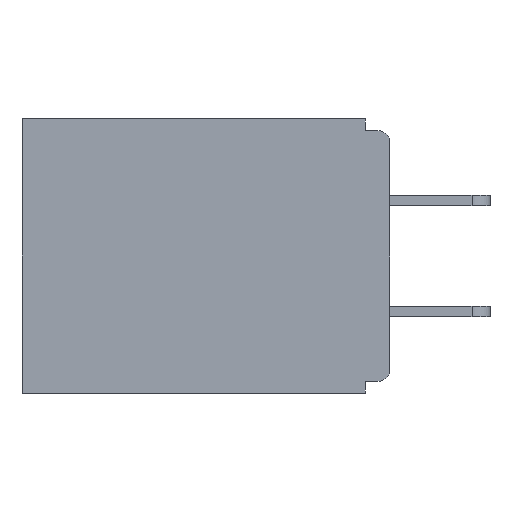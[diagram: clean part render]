
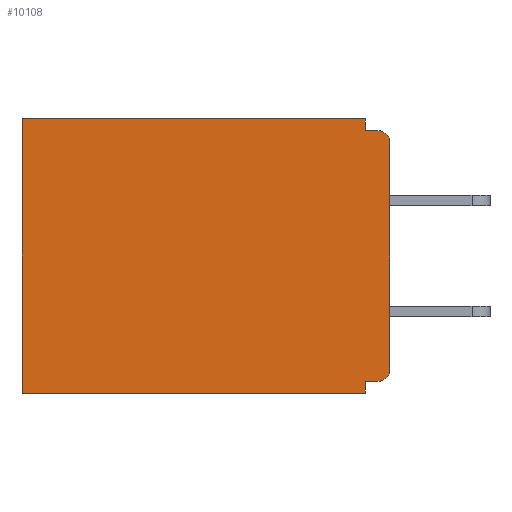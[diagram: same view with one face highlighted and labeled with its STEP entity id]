
A CAD part, left-side view. The second image highlights one B-rep face of the part: STEP entity #10108.
In plain terms, the highlighted planar face has unit normal (-1, 0, 0).
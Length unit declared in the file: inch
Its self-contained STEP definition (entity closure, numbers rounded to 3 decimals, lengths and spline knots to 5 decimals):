
#109 = VERTEX_POINT ( 'NONE', #1873 ) ;
#428 = ORIENTED_EDGE ( 'NONE', *, *, #12479, .F. ) ;
#603 = CARTESIAN_POINT ( 'NONE',  ( 0.298, 0.015, -0.313 ) ) ;
#623 = LINE ( 'NONE', #15823, #2158 ) ;
#644 = LINE ( 'NONE', #12943, #10087 ) ;
#671 = CARTESIAN_POINT ( 'NONE',  ( 0.298, 0.015, -0.015 ) ) ;
#1138 = DIRECTION ( 'NONE',  ( 0., 0., -1. ) ) ;
#1159 = DIRECTION ( 'NONE',  ( 0., 1., 0. ) ) ;
#1163 = VERTEX_POINT ( 'NONE', #1696 ) ;
#1213 = CARTESIAN_POINT ( 'NONE',  ( 0.298, 0., -0.328 ) ) ;
#1373 = VERTEX_POINT ( 'NONE', #3288 ) ;
#1416 = EDGE_CURVE ( 'NONE', #12056, #1445, #12308, .T. ) ;
#1445 = VERTEX_POINT ( 'NONE', #14474 ) ;
#1696 = CARTESIAN_POINT ( 'NONE',  ( 0.298, 0.031, -0.328 ) ) ;
#1727 = DIRECTION ( 'NONE',  ( 0., -1., 0. ) ) ;
#1795 = ORIENTED_EDGE ( 'NONE', *, *, #8183, .F. ) ;
#1815 = VECTOR ( 'NONE', #4954, 39.37008 ) ;
#1835 = LINE ( 'NONE', #6711, #13068 ) ;
#1873 = CARTESIAN_POINT ( 'NONE',  ( 0.298, 0.46, -0.343 ) ) ;
#2158 = VECTOR ( 'NONE', #14056, 39.37008 ) ;
#2245 = DIRECTION ( 'NONE',  ( 0., 0., -1. ) ) ;
#2521 = ORIENTED_EDGE ( 'NONE', *, *, #8639, .T. ) ;
#3025 = LINE ( 'NONE', #12281, #6350 ) ;
#3256 = LINE ( 'NONE', #7422, #12348 ) ;
#3288 = CARTESIAN_POINT ( 'NONE',  ( 0.298, 0.031, -0.015 ) ) ;
#3484 = CARTESIAN_POINT ( 'NONE',  ( 0.298, 0.015, -0.328 ) ) ;
#4926 = CARTESIAN_POINT ( 'NONE',  ( 0.298, 0.031, 0. ) ) ;
#4954 = DIRECTION ( 'NONE',  ( 0., 1., 0. ) ) ;
#5056 = VERTEX_POINT ( 'NONE', #15308 ) ;
#5442 = CARTESIAN_POINT ( 'NONE',  ( 0.298, 0.46, 0. ) ) ;
#5462 = ORIENTED_EDGE ( 'NONE', *, *, #12896, .F. ) ;
#5669 = EDGE_CURVE ( 'NONE', #13512, #1445, #3256, .T. ) ;
#5830 = DIRECTION ( 'NONE',  ( 0., 1., 0. ) ) ;
#6000 = DIRECTION ( 'NONE',  ( -1., 0., 0. ) ) ;
#6046 = AXIS2_PLACEMENT_3D ( 'NONE', #603, #9306, #13221 ) ;
#6350 = VECTOR ( 'NONE', #2245, 39.37008 ) ;
#6384 = AXIS2_PLACEMENT_3D ( 'NONE', #14860, #15900, #8569 ) ;
#6418 = ORIENTED_EDGE ( 'NONE', *, *, #7028, .F. ) ;
#6711 = CARTESIAN_POINT ( 'NONE',  ( 0.298, 0., -0.015 ) ) ;
#7028 = EDGE_CURVE ( 'NONE', #10719, #1373, #3025, .T. ) ;
#7046 = EDGE_LOOP ( 'NONE', ( #9855, #1795, #6418, #2521, #9861, #428, #12510, #5462, #11196, #9612 ) ) ;
#7422 = CARTESIAN_POINT ( 'NONE',  ( 0.298, 0., 0. ) ) ;
#7635 = CIRCLE ( 'NONE', #15856, 0.015 ) ;
#8183 = EDGE_CURVE ( 'NONE', #1373, #9419, #1835, .T. ) ;
#8259 = CARTESIAN_POINT ( 'NONE',  ( 0.298, 0., -0.343 ) ) ;
#8569 = DIRECTION ( 'NONE',  ( 0., 0., -1. ) ) ;
#8623 = VECTOR ( 'NONE', #5830, 39.37008 ) ;
#8639 = EDGE_CURVE ( 'NONE', #10719, #10470, #15396, .T. ) ;
#9102 = EDGE_CURVE ( 'NONE', #1163, #5056, #644, .T. ) ;
#9306 = DIRECTION ( 'NONE',  ( -1., 0., 0. ) ) ;
#9384 = VECTOR ( 'NONE', #1159, 39.37008 ) ;
#9419 = VERTEX_POINT ( 'NONE', #671 ) ;
#9420 = LINE ( 'NONE', #8259, #8623 ) ;
#9612 = ORIENTED_EDGE ( 'NONE', *, *, #5669, .F. ) ;
#9855 = ORIENTED_EDGE ( 'NONE', *, *, #12700, .T. ) ;
#9861 = ORIENTED_EDGE ( 'NONE', *, *, #11090, .T. ) ;
#10087 = VECTOR ( 'NONE', #14303, 39.37008 ) ;
#10108 = ADVANCED_FACE ( 'NONE', ( #14792 ), #13600, .F. ) ;
#10470 = VERTEX_POINT ( 'NONE', #5442 ) ;
#10719 = VERTEX_POINT ( 'NONE', #4926 ) ;
#11090 = EDGE_CURVE ( 'NONE', #10470, #109, #623, .T. ) ;
#11112 = CARTESIAN_POINT ( 'NONE',  ( 0.298, 0.015, -0.03 ) ) ;
#11196 = ORIENTED_EDGE ( 'NONE', *, *, #1416, .T. ) ;
#12056 = VERTEX_POINT ( 'NONE', #3484 ) ;
#12281 = CARTESIAN_POINT ( 'NONE',  ( 0.298, 0.031, -0.343 ) ) ;
#12308 = CIRCLE ( 'NONE', #6046, 0.015 ) ;
#12348 = VECTOR ( 'NONE', #16180, 39.37008 ) ;
#12479 = EDGE_CURVE ( 'NONE', #5056, #109, #9420, .T. ) ;
#12509 = CARTESIAN_POINT ( 'NONE',  ( 0.298, 0., 0. ) ) ;
#12510 = ORIENTED_EDGE ( 'NONE', *, *, #9102, .F. ) ;
#12700 = EDGE_CURVE ( 'NONE', #13512, #9419, #7635, .T. ) ;
#12759 = LINE ( 'NONE', #1213, #9384 ) ;
#12896 = EDGE_CURVE ( 'NONE', #12056, #1163, #12759, .T. ) ;
#12943 = CARTESIAN_POINT ( 'NONE',  ( 0.298, 0.031, -0.343 ) ) ;
#13068 = VECTOR ( 'NONE', #1727, 39.37008 ) ;
#13221 = DIRECTION ( 'NONE',  ( 0., 0., -1. ) ) ;
#13512 = VERTEX_POINT ( 'NONE', #15680 ) ;
#13600 = PLANE ( 'NONE',  #6384 ) ;
#14056 = DIRECTION ( 'NONE',  ( 0., 0., -1. ) ) ;
#14303 = DIRECTION ( 'NONE',  ( 0., 0., -1. ) ) ;
#14474 = CARTESIAN_POINT ( 'NONE',  ( 0.298, 0., -0.313 ) ) ;
#14792 = FACE_OUTER_BOUND ( 'NONE', #7046, .T. ) ;
#14860 = CARTESIAN_POINT ( 'NONE',  ( 0.298, 0., 0. ) ) ;
#15308 = CARTESIAN_POINT ( 'NONE',  ( 0.298, 0.031, -0.343 ) ) ;
#15396 = LINE ( 'NONE', #12509, #1815 ) ;
#15680 = CARTESIAN_POINT ( 'NONE',  ( 0.298, 0., -0.03 ) ) ;
#15823 = CARTESIAN_POINT ( 'NONE',  ( 0.298, 0.46, 0. ) ) ;
#15856 = AXIS2_PLACEMENT_3D ( 'NONE', #11112, #6000, #1138 ) ;
#15900 = DIRECTION ( 'NONE',  ( 1., 0., 0. ) ) ;
#16180 = DIRECTION ( 'NONE',  ( 0., 0., -1. ) ) ;
